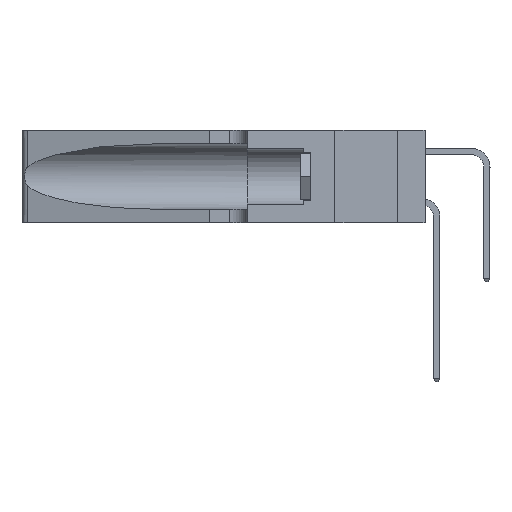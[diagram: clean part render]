
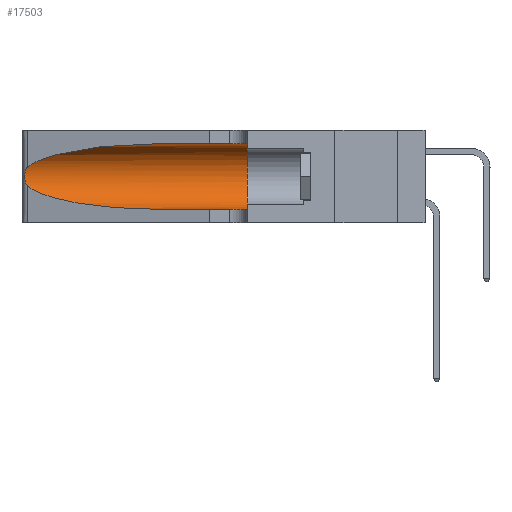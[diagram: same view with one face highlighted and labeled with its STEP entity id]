
A CAD part, left-side view. The second image highlights one B-rep face of the part: STEP entity #17503.
In plain terms, the highlighted cylindrical face has radius 3.308 mm (diameter 6.617 mm), a partial arc.
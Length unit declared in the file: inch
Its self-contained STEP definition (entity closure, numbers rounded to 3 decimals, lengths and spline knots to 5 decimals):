
#614 = B_SPLINE_CURVE_WITH_KNOTS ( 'NONE', 3,
 ( #17471, #11255, #14352, #20611, #7841, #12863, #6165, #11187, #3283, #17610, #6300, #7984, #1619, #3018 ),
 .UNSPECIFIED., .F., .F.,
 ( 4, 2, 2, 2, 2, 2, 4 ),
 ( 0., 0.00027, 0.00053, 0.00107, 0.0016, 0.00187, 0.00214 ),
 .UNSPECIFIED. ) ;
#658 = CARTESIAN_POINT ( 'NONE',  ( 0.1305, 0.72297, 0.31525 ) ) ;
#911 = CARTESIAN_POINT ( 'NONE',  ( 0.1305, 1.61858, 0.31525 ) ) ;
#1492 = ORIENTED_EDGE ( 'NONE', *, *, #16446, .T. ) ;
#1619 = CARTESIAN_POINT ( 'NONE',  ( 0.25555, 1.22993, 0.14849 ) ) ;
#1822 = CARTESIAN_POINT ( 'NONE',  ( 0.25487, 1.22718, 0.22369 ) ) ;
#2244 = CARTESIAN_POINT ( 'NONE',  ( 0.18966, 0.96281, 0.31525 ) ) ;
#2270 = ORIENTED_EDGE ( 'NONE', *, *, #10830, .F. ) ;
#2815 = VERTEX_POINT ( 'NONE', #3096 ) ;
#3018 = CARTESIAN_POINT ( 'NONE',  ( 0.25487, 1.22718, 0.14631 ) ) ;
#3019 = ORIENTED_EDGE ( 'NONE', *, *, #12703, .T. ) ;
#3096 = CARTESIAN_POINT ( 'NONE',  ( 0.1305, 0.35, 0.05475 ) ) ;
#3283 = CARTESIAN_POINT ( 'NONE',  ( 0.26017, 1.23833, 0.17102 ) ) ;
#3537 = CARTESIAN_POINT ( 'NONE',  ( 0.1305, 1.61858, 0.185 ) ) ;
#3549 = CARTESIAN_POINT ( 'NONE',  ( 0.1305, 0.35, 0.31525 ) ) ;
#3859 = CARTESIAN_POINT ( 'NONE',  ( 0.25487, 1.22718, 0.22369 ) ) ;
#4302 = CARTESIAN_POINT ( 'NONE',  ( 0.25487, 1.22718, 0.14631 ) ) ;
#4680 = VERTEX_POINT ( 'NONE', #15626 ) ;
#4691 = EDGE_LOOP ( 'NONE', ( #1492, #16430, #12343, #3019, #2270, #16178 ) ) ;
#4885 = VECTOR ( 'NONE', #15308, 39.37008 ) ;
#4941 = VERTEX_POINT ( 'NONE', #4302 ) ;
#4952 =( BOUNDED_CURVE ( )  B_SPLINE_CURVE ( 3, ( #17392, #17321, #5041, #12917 ),
 .UNSPECIFIED., .F., .T. ) 
 B_SPLINE_CURVE_WITH_KNOTS ( ( 4, 4 ),
 ( 3.44316, 4.71239 ),
 .UNSPECIFIED. ) 
 CURVE ( )  GEOMETRIC_REPRESENTATION_ITEM ( )  RATIONAL_B_SPLINE_CURVE ( ( 1., 0.87, 0.87, 1. ) ) 
 REPRESENTATION_ITEM ( '' )  );
#5041 = CARTESIAN_POINT ( 'NONE',  ( 0.18966, 0.96281, 0.05475 ) ) ;
#5449 = CARTESIAN_POINT ( 'NONE',  ( 0.2373, 1.15595, 0.28018 ) ) ;
#5893 = VERTEX_POINT ( 'NONE', #3549 ) ;
#6165 = CARTESIAN_POINT ( 'NONE',  ( 0.26075, 1.23896, 0.19203 ) ) ;
#6300 = CARTESIAN_POINT ( 'NONE',  ( 0.25789, 1.23486, 0.15765 ) ) ;
#6878 = DIRECTION ( 'NONE',  ( 0., 0., 1. ) ) ;
#6908 = DIRECTION ( 'NONE',  ( 0., -1., 0. ) ) ;
#7094 = CARTESIAN_POINT ( 'NONE',  ( 0.1305, 0.72297, 0.05475 ) ) ;
#7687 = EDGE_CURVE ( 'NONE', #4680, #5893, #13609, .T. ) ;
#7841 = CARTESIAN_POINT ( 'NONE',  ( 0.25854, 1.2359, 0.20912 ) ) ;
#7984 = CARTESIAN_POINT ( 'NONE',  ( 0.25639, 1.23186, 0.15144 ) ) ;
#8234 = CARTESIAN_POINT ( 'NONE',  ( 0.1305, 0.35, 0.185 ) ) ;
#8820 = LINE ( 'NONE', #16905, #9832 ) ;
#8933 = AXIS2_PLACEMENT_3D ( 'NONE', #3537, #6908, #14932 ) ;
#9013 =( BOUNDED_CURVE ( )  B_SPLINE_CURVE ( 3, ( #658, #2244, #5449, #3859 ),
 .UNSPECIFIED., .F., .F. ) 
 B_SPLINE_CURVE_WITH_KNOTS ( ( 4, 4 ),
 ( 1.5708, 2.84003 ),
 .UNSPECIFIED. ) 
 CURVE ( )  GEOMETRIC_REPRESENTATION_ITEM ( )  RATIONAL_B_SPLINE_CURVE ( ( 1., 0.87, 0.87, 1. ) ) 
 REPRESENTATION_ITEM ( '' )  );
#9832 = VECTOR ( 'NONE', #9881, 39.37008 ) ;
#9881 = DIRECTION ( 'NONE',  ( 0., -1., 0. ) ) ;
#10830 = EDGE_CURVE ( 'NONE', #5893, #2815, #19404, .T. ) ;
#11187 = CARTESIAN_POINT ( 'NONE',  ( 0.26075, 1.23896, 0.178 ) ) ;
#11200 = EDGE_CURVE ( 'NONE', #4941, #15768, #4952, .T. ) ;
#11255 = CARTESIAN_POINT ( 'NONE',  ( 0.25555, 1.22994, 0.2215 ) ) ;
#12343 = ORIENTED_EDGE ( 'NONE', *, *, #11200, .T. ) ;
#12703 = EDGE_CURVE ( 'NONE', #15768, #2815, #8820, .T. ) ;
#12739 = AXIS2_PLACEMENT_3D ( 'NONE', #8234, #14770, #6878 ) ;
#12863 = CARTESIAN_POINT ( 'NONE',  ( 0.26018, 1.23835, 0.19895 ) ) ;
#12917 = CARTESIAN_POINT ( 'NONE',  ( 0.1305, 0.72297, 0.05475 ) ) ;
#13609 = LINE ( 'NONE', #911, #4885 ) ;
#14352 = CARTESIAN_POINT ( 'NONE',  ( 0.25639, 1.23184, 0.21858 ) ) ;
#14770 = DIRECTION ( 'NONE',  ( 0., 1., 0. ) ) ;
#14932 = DIRECTION ( 'NONE',  ( 0., 0., -1. ) ) ;
#15251 = FACE_OUTER_BOUND ( 'NONE', #4691, .T. ) ;
#15308 = DIRECTION ( 'NONE',  ( 0., -1., 0. ) ) ;
#15626 = CARTESIAN_POINT ( 'NONE',  ( 0.1305, 0.72297, 0.31525 ) ) ;
#15768 = VERTEX_POINT ( 'NONE', #7094 ) ;
#16087 = EDGE_CURVE ( 'NONE', #19395, #4941, #614, .T. ) ;
#16178 = ORIENTED_EDGE ( 'NONE', *, *, #7687, .F. ) ;
#16430 = ORIENTED_EDGE ( 'NONE', *, *, #16087, .T. ) ;
#16446 = EDGE_CURVE ( 'NONE', #4680, #19395, #9013, .T. ) ;
#16905 = CARTESIAN_POINT ( 'NONE',  ( 0.1305, 1.61858, 0.05475 ) ) ;
#17321 = CARTESIAN_POINT ( 'NONE',  ( 0.2373, 1.15595, 0.08982 ) ) ;
#17392 = CARTESIAN_POINT ( 'NONE',  ( 0.25487, 1.22718, 0.14631 ) ) ;
#17471 = CARTESIAN_POINT ( 'NONE',  ( 0.25487, 1.22718, 0.22369 ) ) ;
#17503 = ADVANCED_FACE ( 'NONE', ( #15251 ), #18476, .F. ) ;
#17610 = CARTESIAN_POINT ( 'NONE',  ( 0.25856, 1.23593, 0.16098 ) ) ;
#18476 = CYLINDRICAL_SURFACE ( 'NONE', #8933, 0.13025 ) ;
#19395 = VERTEX_POINT ( 'NONE', #1822 ) ;
#19404 = CIRCLE ( 'NONE', #12739, 0.13025 ) ;
#20611 = CARTESIAN_POINT ( 'NONE',  ( 0.25787, 1.23484, 0.2124 ) ) ;
